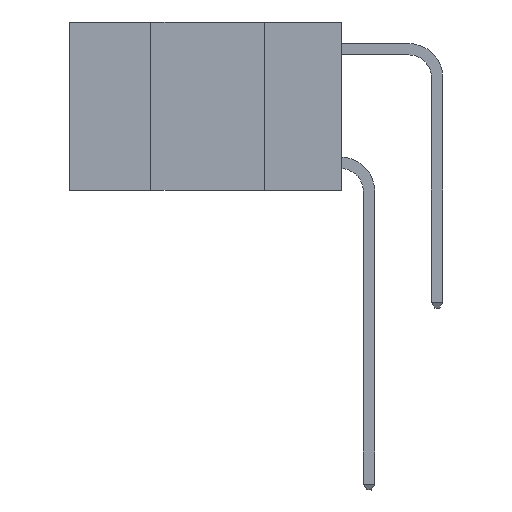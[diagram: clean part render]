
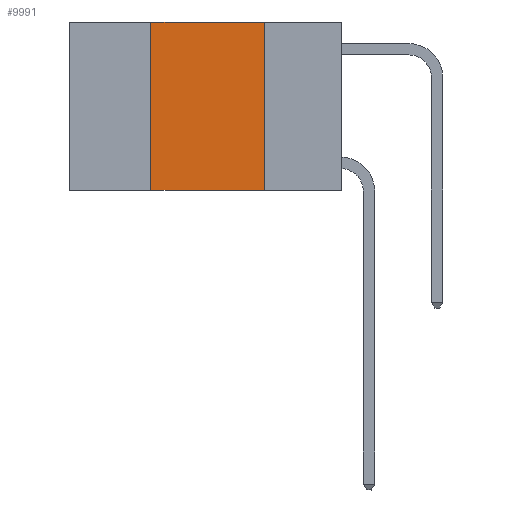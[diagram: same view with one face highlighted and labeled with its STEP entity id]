
A CAD part, left-side view. The second image highlights one B-rep face of the part: STEP entity #9991.
In plain terms, the highlighted planar face has unit normal (-1, 0, 0).
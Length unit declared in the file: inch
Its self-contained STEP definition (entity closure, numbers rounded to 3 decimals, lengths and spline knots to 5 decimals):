
#160 = EDGE_CURVE ( 'NONE', #4150, #9601, #2798, .T. ) ;
#1004 = DIRECTION ( 'NONE',  ( 0., -1., 0. ) ) ;
#2332 = PLANE ( 'NONE',  #10793 ) ;
#2484 = VERTEX_POINT ( 'NONE', #6882 ) ;
#2651 = CARTESIAN_POINT ( 'NONE',  ( 0., 0.17, 0. ) ) ;
#2682 = CARTESIAN_POINT ( 'NONE',  ( 0., 0.42, 0. ) ) ;
#2798 = LINE ( 'NONE', #8812, #9299 ) ;
#2887 = DIRECTION ( 'NONE',  ( 0., 0., 1. ) ) ;
#3356 = EDGE_LOOP ( 'NONE', ( #3656, #8654, #8307, #8117 ) ) ;
#3400 = LINE ( 'NONE', #7897, #12975 ) ;
#3480 = CARTESIAN_POINT ( 'NONE',  ( 0., 0.6, 0. ) ) ;
#3633 = EDGE_CURVE ( 'NONE', #4150, #4658, #3400, .T. ) ;
#3656 = ORIENTED_EDGE ( 'NONE', *, *, #4298, .F. ) ;
#4150 = VERTEX_POINT ( 'NONE', #6011 ) ;
#4298 = EDGE_CURVE ( 'NONE', #2484, #4658, #13316, .T. ) ;
#4658 = VERTEX_POINT ( 'NONE', #12572 ) ;
#6011 = CARTESIAN_POINT ( 'NONE',  ( 0., 0.42, -0.37 ) ) ;
#6210 = DIRECTION ( 'NONE',  ( 0., 0., -1. ) ) ;
#6552 = FACE_OUTER_BOUND ( 'NONE', #3356, .T. ) ;
#6882 = CARTESIAN_POINT ( 'NONE',  ( 0., 0.17, 0. ) ) ;
#7897 = CARTESIAN_POINT ( 'NONE',  ( 0., 0.6, -0.37 ) ) ;
#8117 = ORIENTED_EDGE ( 'NONE', *, *, #3633, .T. ) ;
#8307 = ORIENTED_EDGE ( 'NONE', *, *, #160, .F. ) ;
#8654 = ORIENTED_EDGE ( 'NONE', *, *, #9122, .F. ) ;
#8812 = CARTESIAN_POINT ( 'NONE',  ( 0., 0.42, 0. ) ) ;
#9122 = EDGE_CURVE ( 'NONE', #9601, #2484, #12881, .T. ) ;
#9299 = VECTOR ( 'NONE', #2887, 39.37008 ) ;
#9601 = VERTEX_POINT ( 'NONE', #2682 ) ;
#9991 = ADVANCED_FACE ( 'NONE', ( #6552 ), #2332, .F. ) ;
#10167 = VECTOR ( 'NONE', #12458, 39.37008 ) ;
#10241 = VECTOR ( 'NONE', #6210, 39.37008 ) ;
#10793 = AXIS2_PLACEMENT_3D ( 'NONE', #3480, #13928, #14964 ) ;
#12458 = DIRECTION ( 'NONE',  ( 0., -1., 0. ) ) ;
#12572 = CARTESIAN_POINT ( 'NONE',  ( 0., 0.17, -0.37 ) ) ;
#12881 = LINE ( 'NONE', #13510, #10167 ) ;
#12975 = VECTOR ( 'NONE', #1004, 39.37008 ) ;
#13316 = LINE ( 'NONE', #2651, #10241 ) ;
#13510 = CARTESIAN_POINT ( 'NONE',  ( 0., 0.6, 0. ) ) ;
#13928 = DIRECTION ( 'NONE',  ( 1., 0., 0. ) ) ;
#14964 = DIRECTION ( 'NONE',  ( 0., 0., -1. ) ) ;
